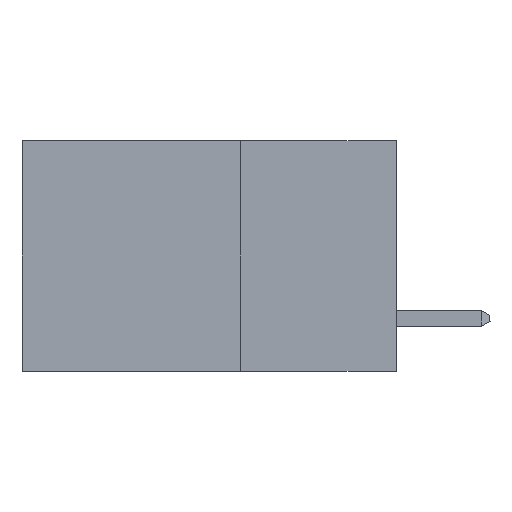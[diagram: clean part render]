
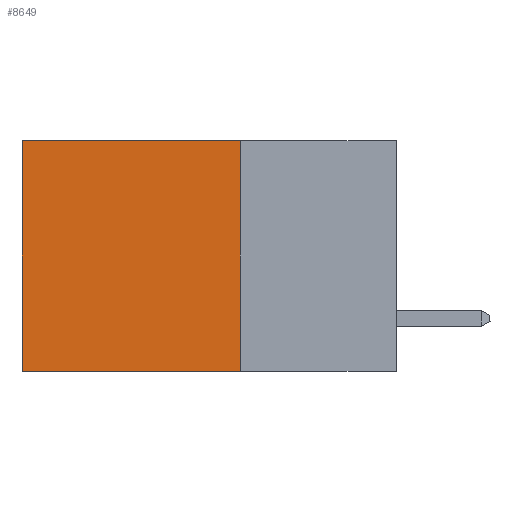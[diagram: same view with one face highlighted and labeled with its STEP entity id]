
A CAD part, left-side view. The second image highlights one B-rep face of the part: STEP entity #8649.
In plain terms, the highlighted planar face has unit normal (-1, 0, 0).
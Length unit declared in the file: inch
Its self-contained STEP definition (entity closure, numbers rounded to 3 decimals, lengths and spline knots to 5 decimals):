
#235 = AXIS2_PLACEMENT_3D ( 'NONE', #4676, #5627, #4791 ) ;
#1302 = CARTESIAN_POINT ( 'NONE',  ( 0.298, 0.6, -0.37 ) ) ;
#1812 = FACE_OUTER_BOUND ( 'NONE', #6300, .T. ) ;
#2268 = LINE ( 'NONE', #7559, #4086 ) ;
#2717 = DIRECTION ( 'NONE',  ( 0., 0., -1. ) ) ;
#2980 = DIRECTION ( 'NONE',  ( 0., 0., -1. ) ) ;
#3081 = VERTEX_POINT ( 'NONE', #7468 ) ;
#3094 = CARTESIAN_POINT ( 'NONE',  ( 0.298, 0.25, 0. ) ) ;
#3437 = VERTEX_POINT ( 'NONE', #1302 ) ;
#3843 = ORIENTED_EDGE ( 'NONE', *, *, #10306, .T. ) ;
#4086 = VECTOR ( 'NONE', #10275, 39.37008 ) ;
#4220 = CARTESIAN_POINT ( 'NONE',  ( 0.298, 0.25, -0.37 ) ) ;
#4416 = VERTEX_POINT ( 'NONE', #3094 ) ;
#4676 = CARTESIAN_POINT ( 'NONE',  ( 0.298, 0.25, 0. ) ) ;
#4791 = DIRECTION ( 'NONE',  ( 0., 0., -1. ) ) ;
#5085 = LINE ( 'NONE', #6505, #6734 ) ;
#5271 = VECTOR ( 'NONE', #2717, 39.37008 ) ;
#5400 = CARTESIAN_POINT ( 'NONE',  ( 0.298, 0.25, -0.37 ) ) ;
#5599 = EDGE_CURVE ( 'NONE', #3081, #3437, #5085, .T. ) ;
#5616 = ORIENTED_EDGE ( 'NONE', *, *, #10399, .F. ) ;
#5627 = DIRECTION ( 'NONE',  ( 1., 0., 0. ) ) ;
#6300 = EDGE_LOOP ( 'NONE', ( #9311, #5616, #9105, #3843 ) ) ;
#6435 = VERTEX_POINT ( 'NONE', #5400 ) ;
#6505 = CARTESIAN_POINT ( 'NONE',  ( 0.298, 0.6, 0. ) ) ;
#6734 = VECTOR ( 'NONE', #2980, 39.37008 ) ;
#6944 = LINE ( 'NONE', #8948, #5271 ) ;
#7468 = CARTESIAN_POINT ( 'NONE',  ( 0.298, 0.6, 0. ) ) ;
#7559 = CARTESIAN_POINT ( 'NONE',  ( 0.298, 0.25, 0. ) ) ;
#8339 = VECTOR ( 'NONE', #11342, 39.37008 ) ;
#8541 = PLANE ( 'NONE',  #235 ) ;
#8649 = ADVANCED_FACE ( 'NONE', ( #1812 ), #8541, .F. ) ;
#8774 = LINE ( 'NONE', #4220, #8339 ) ;
#8948 = CARTESIAN_POINT ( 'NONE',  ( 0.298, 0.25, 0. ) ) ;
#9105 = ORIENTED_EDGE ( 'NONE', *, *, #9585, .F. ) ;
#9311 = ORIENTED_EDGE ( 'NONE', *, *, #5599, .T. ) ;
#9585 = EDGE_CURVE ( 'NONE', #4416, #6435, #6944, .T. ) ;
#10275 = DIRECTION ( 'NONE',  ( 0., 1., 0. ) ) ;
#10306 = EDGE_CURVE ( 'NONE', #4416, #3081, #2268, .T. ) ;
#10399 = EDGE_CURVE ( 'NONE', #6435, #3437, #8774, .T. ) ;
#11342 = DIRECTION ( 'NONE',  ( 0., 1., 0. ) ) ;
